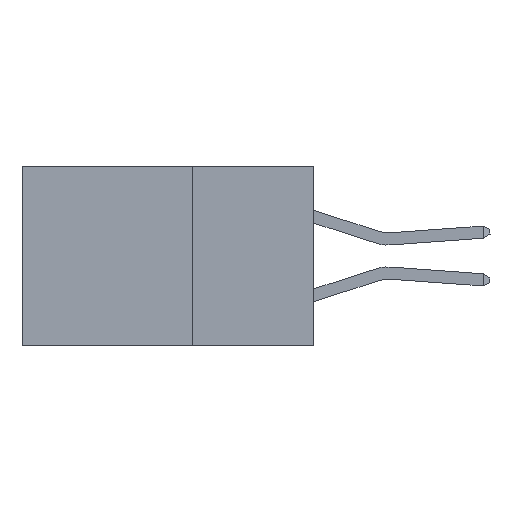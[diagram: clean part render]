
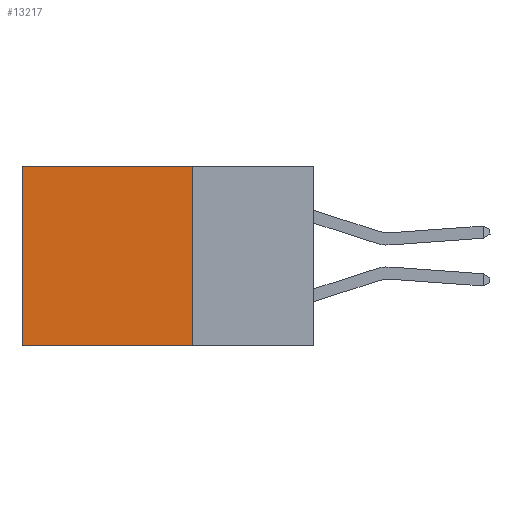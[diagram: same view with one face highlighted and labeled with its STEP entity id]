
A CAD part, left-side view. The second image highlights one B-rep face of the part: STEP entity #13217.
In plain terms, the highlighted planar face has unit normal (-1, 0, 0).
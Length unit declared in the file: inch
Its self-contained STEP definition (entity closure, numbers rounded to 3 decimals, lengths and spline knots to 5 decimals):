
#353 = DIRECTION ( 'NONE',  ( 1., 0., 0. ) ) ;
#1812 = LINE ( 'NONE', #11743, #5022 ) ;
#2502 = VERTEX_POINT ( 'NONE', #4500 ) ;
#2717 = VERTEX_POINT ( 'NONE', #17190 ) ;
#3173 = DIRECTION ( 'NONE',  ( 0., 1., 0. ) ) ;
#3584 = VECTOR ( 'NONE', #20448, 39.37008 ) ;
#3659 = FACE_OUTER_BOUND ( 'NONE', #10641, .T. ) ;
#4500 = CARTESIAN_POINT ( 'NONE',  ( 0.2875, 0.6, 0. ) ) ;
#4573 = CARTESIAN_POINT ( 'NONE',  ( 0.2875, 0.25, 0. ) ) ;
#5022 = VECTOR ( 'NONE', #18480, 39.37008 ) ;
#5188 = DIRECTION ( 'NONE',  ( 0., 0., -1. ) ) ;
#5316 = LINE ( 'NONE', #12051, #6601 ) ;
#5724 = EDGE_CURVE ( 'NONE', #19067, #2502, #15487, .T. ) ;
#6601 = VECTOR ( 'NONE', #18782, 39.37008 ) ;
#8413 = CARTESIAN_POINT ( 'NONE',  ( 0.2875, 0.25, 0. ) ) ;
#8650 = CARTESIAN_POINT ( 'NONE',  ( 0.2875, 0.6, -0.37 ) ) ;
#9639 = EDGE_CURVE ( 'NONE', #2717, #11068, #13645, .T. ) ;
#10641 = EDGE_LOOP ( 'NONE', ( #18919, #11642, #17162, #20843 ) ) ;
#11068 = VERTEX_POINT ( 'NONE', #8650 ) ;
#11642 = ORIENTED_EDGE ( 'NONE', *, *, #9639, .F. ) ;
#11710 = CARTESIAN_POINT ( 'NONE',  ( 0.2875, 0.25, 0. ) ) ;
#11743 = CARTESIAN_POINT ( 'NONE',  ( 0.2875, 0.25, 0. ) ) ;
#11887 = CARTESIAN_POINT ( 'NONE',  ( 0.2875, 0.25, -0.37 ) ) ;
#12051 = CARTESIAN_POINT ( 'NONE',  ( 0.2875, 0.6, 0. ) ) ;
#13217 = ADVANCED_FACE ( 'NONE', ( #3659 ), #16778, .F. ) ;
#13645 = LINE ( 'NONE', #11887, #15757 ) ;
#15487 = LINE ( 'NONE', #8413, #3584 ) ;
#15757 = VECTOR ( 'NONE', #3173, 39.37008 ) ;
#16778 = PLANE ( 'NONE',  #20423 ) ;
#16975 = EDGE_CURVE ( 'NONE', #19067, #2717, #1812, .T. ) ;
#17162 = ORIENTED_EDGE ( 'NONE', *, *, #16975, .F. ) ;
#17190 = CARTESIAN_POINT ( 'NONE',  ( 0.2875, 0.25, -0.37 ) ) ;
#18480 = DIRECTION ( 'NONE',  ( 0., 0., -1. ) ) ;
#18782 = DIRECTION ( 'NONE',  ( 0., 0., -1. ) ) ;
#18919 = ORIENTED_EDGE ( 'NONE', *, *, #19974, .T. ) ;
#19067 = VERTEX_POINT ( 'NONE', #4573 ) ;
#19974 = EDGE_CURVE ( 'NONE', #2502, #11068, #5316, .T. ) ;
#20423 = AXIS2_PLACEMENT_3D ( 'NONE', #11710, #353, #5188 ) ;
#20448 = DIRECTION ( 'NONE',  ( 0., 1., 0. ) ) ;
#20843 = ORIENTED_EDGE ( 'NONE', *, *, #5724, .T. ) ;
